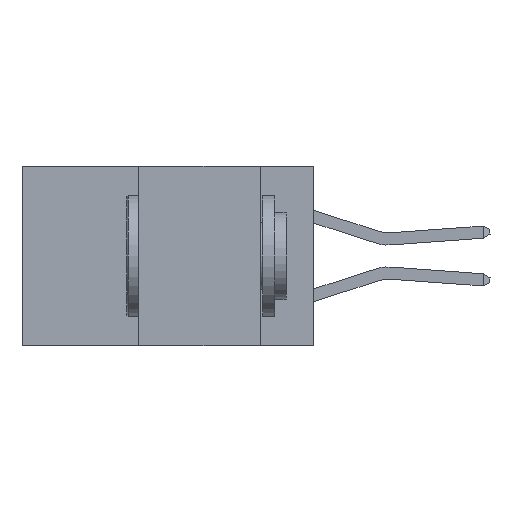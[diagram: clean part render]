
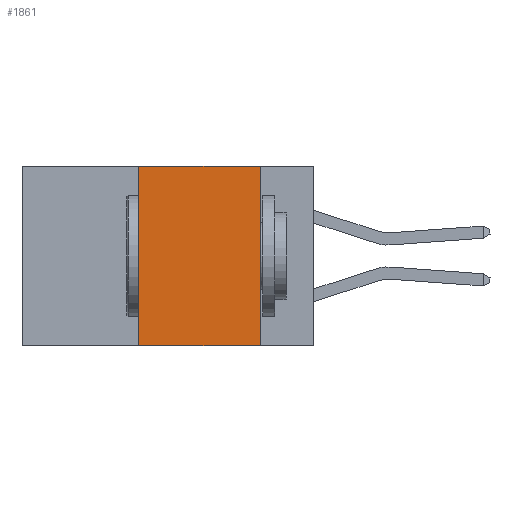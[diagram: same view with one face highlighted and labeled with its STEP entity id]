
A CAD part, left-side view. The second image highlights one B-rep face of the part: STEP entity #1861.
In plain terms, the highlighted planar face has unit normal (-1, 0, 0).
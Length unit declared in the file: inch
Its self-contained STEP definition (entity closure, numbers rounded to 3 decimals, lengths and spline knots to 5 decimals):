
#409 = FACE_OUTER_BOUND ( 'NONE', #3384, .T. ) ;
#796 = LINE ( 'NONE', #1897, #17951 ) ;
#1861 = ADVANCED_FACE ( 'NONE', ( #409 ), #2756, .F. ) ;
#1890 = DIRECTION ( 'NONE',  ( 0., -1., 0. ) ) ;
#1897 = CARTESIAN_POINT ( 'NONE',  ( 0., 0.6, 0. ) ) ;
#2054 = ORIENTED_EDGE ( 'NONE', *, *, #4757, .T. ) ;
#2374 = LINE ( 'NONE', #9959, #11692 ) ;
#2756 = PLANE ( 'NONE',  #17558 ) ;
#2833 = DIRECTION ( 'NONE',  ( 1., 0., 0. ) ) ;
#3384 = EDGE_LOOP ( 'NONE', ( #20385, #5352, #11383, #2054 ) ) ;
#4162 = DIRECTION ( 'NONE',  ( 0., 0., 1. ) ) ;
#4757 = EDGE_CURVE ( 'NONE', #9462, #14738, #8755, .T. ) ;
#5242 = CARTESIAN_POINT ( 'NONE',  ( 0., 0.6, -0.37 ) ) ;
#5352 = ORIENTED_EDGE ( 'NONE', *, *, #14270, .F. ) ;
#5534 = CARTESIAN_POINT ( 'NONE',  ( 0., 0.36, 0. ) ) ;
#8141 = VERTEX_POINT ( 'NONE', #10177 ) ;
#8755 = LINE ( 'NONE', #5242, #10855 ) ;
#9462 = VERTEX_POINT ( 'NONE', #10444 ) ;
#9959 = CARTESIAN_POINT ( 'NONE',  ( 0., 0.11, 0. ) ) ;
#10177 = CARTESIAN_POINT ( 'NONE',  ( 0., 0.36, 0. ) ) ;
#10444 = CARTESIAN_POINT ( 'NONE',  ( 0., 0.36, -0.37 ) ) ;
#10855 = VECTOR ( 'NONE', #1890, 39.37008 ) ;
#11383 = ORIENTED_EDGE ( 'NONE', *, *, #16287, .F. ) ;
#11594 = CARTESIAN_POINT ( 'NONE',  ( 0., 0.11, -0.37 ) ) ;
#11692 = VECTOR ( 'NONE', #18748, 39.37008 ) ;
#12975 = CARTESIAN_POINT ( 'NONE',  ( 0., 0.6, 0. ) ) ;
#13379 = EDGE_CURVE ( 'NONE', #13575, #14738, #2374, .T. ) ;
#13571 = DIRECTION ( 'NONE',  ( 0., -1., 0. ) ) ;
#13575 = VERTEX_POINT ( 'NONE', #17407 ) ;
#14270 = EDGE_CURVE ( 'NONE', #8141, #13575, #796, .T. ) ;
#14738 = VERTEX_POINT ( 'NONE', #11594 ) ;
#14970 = LINE ( 'NONE', #5534, #18857 ) ;
#16287 = EDGE_CURVE ( 'NONE', #9462, #8141, #14970, .T. ) ;
#17407 = CARTESIAN_POINT ( 'NONE',  ( 0., 0.11, 0. ) ) ;
#17558 = AXIS2_PLACEMENT_3D ( 'NONE', #12975, #2833, #21364 ) ;
#17951 = VECTOR ( 'NONE', #13571, 39.37008 ) ;
#18748 = DIRECTION ( 'NONE',  ( 0., 0., -1. ) ) ;
#18857 = VECTOR ( 'NONE', #4162, 39.37008 ) ;
#20385 = ORIENTED_EDGE ( 'NONE', *, *, #13379, .F. ) ;
#21364 = DIRECTION ( 'NONE',  ( 0., 0., -1. ) ) ;
